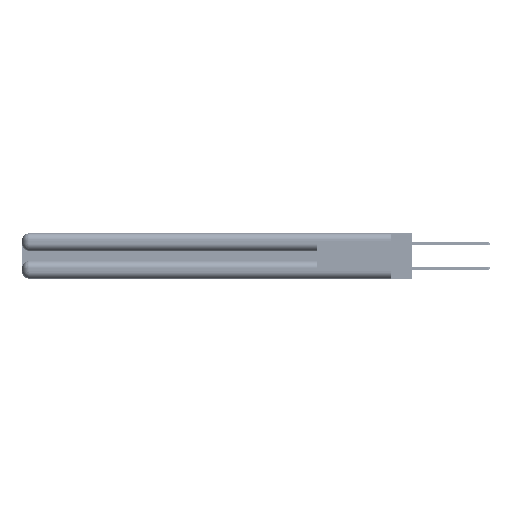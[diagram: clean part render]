
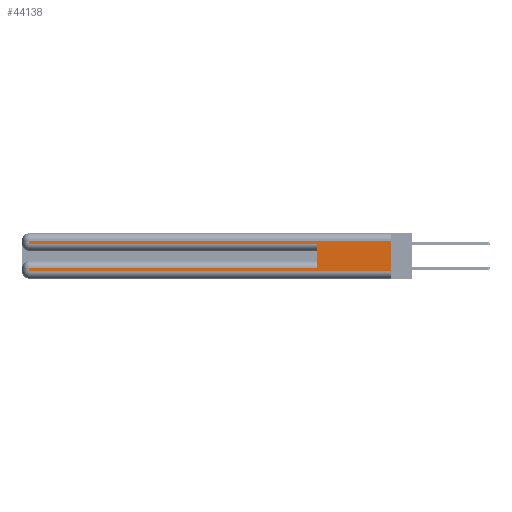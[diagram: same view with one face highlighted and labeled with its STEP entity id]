
A CAD part, left-side view. The second image highlights one B-rep face of the part: STEP entity #44138.
In plain terms, the highlighted planar face has unit normal (-1, 0, 0).
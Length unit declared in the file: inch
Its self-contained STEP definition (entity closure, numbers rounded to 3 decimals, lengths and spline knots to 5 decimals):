
#1636 = CARTESIAN_POINT ( 'NONE',  ( 0., 0., 0.37 ) ) ;
#1816 = CARTESIAN_POINT ( 'NONE',  ( 0., 0., 0.37 ) ) ;
#1879 = VERTEX_POINT ( 'NONE', #38098 ) ;
#2134 = DIRECTION ( 'NONE',  ( 0., 0., -1. ) ) ;
#2666 = ORIENTED_EDGE ( 'NONE', *, *, #47249, .T. ) ;
#5046 = LINE ( 'NONE', #14562, #25604 ) ;
#6629 = DIRECTION ( 'NONE',  ( 0., -1., 0. ) ) ;
#7760 = EDGE_CURVE ( 'NONE', #37095, #1879, #13730, .T. ) ;
#7888 = CARTESIAN_POINT ( 'NONE',  ( 0., 0., 0.06 ) ) ;
#8126 = DIRECTION ( 'NONE',  ( 0., 0., 1. ) ) ;
#9948 = CARTESIAN_POINT ( 'NONE',  ( 0., 2.94, 0.37 ) ) ;
#10549 = CARTESIAN_POINT ( 'NONE',  ( 0., 2.94, 0.31 ) ) ;
#12136 = VECTOR ( 'NONE', #12455, 39.37008 ) ;
#12435 = ORIENTED_EDGE ( 'NONE', *, *, #36582, .T. ) ;
#12455 = DIRECTION ( 'NONE',  ( 0., 1., 0. ) ) ;
#12641 = CARTESIAN_POINT ( 'NONE',  ( 0., 0.6, 0.145 ) ) ;
#13730 = LINE ( 'NONE', #9948, #21388 ) ;
#14257 = DIRECTION ( 'NONE',  ( 0., 0., -1. ) ) ;
#14562 = CARTESIAN_POINT ( 'NONE',  ( 0., 0., 0.06 ) ) ;
#18042 = DIRECTION ( 'NONE',  ( 0., -1., 0. ) ) ;
#18179 = DIRECTION ( 'NONE',  ( 0., 0., -1. ) ) ;
#18964 = CARTESIAN_POINT ( 'NONE',  ( 0., 2.94, 0.285 ) ) ;
#19004 = FACE_OUTER_BOUND ( 'NONE', #50883, .T. ) ;
#21388 = VECTOR ( 'NONE', #18179, 39.37008 ) ;
#21871 = EDGE_CURVE ( 'NONE', #32762, #28467, #35847, .T. ) ;
#23206 = LINE ( 'NONE', #50889, #35406 ) ;
#24456 = VECTOR ( 'NONE', #8126, 39.37008 ) ;
#24737 = VERTEX_POINT ( 'NONE', #26861 ) ;
#25323 = EDGE_CURVE ( 'NONE', #25423, #47871, #34207, .T. ) ;
#25423 = VERTEX_POINT ( 'NONE', #47797 ) ;
#25604 = VECTOR ( 'NONE', #6629, 39.37008 ) ;
#26383 = ORIENTED_EDGE ( 'NONE', *, *, #41433, .F. ) ;
#26861 = CARTESIAN_POINT ( 'NONE',  ( 0., 0.6, 0.085 ) ) ;
#28196 = CARTESIAN_POINT ( 'NONE',  ( 0., 0., 0.31 ) ) ;
#28467 = VERTEX_POINT ( 'NONE', #18964 ) ;
#30364 = DIRECTION ( 'NONE',  ( 0., 0., -1. ) ) ;
#32016 = ORIENTED_EDGE ( 'NONE', *, *, #40939, .T. ) ;
#32537 = DIRECTION ( 'NONE',  ( 0., 1., 0. ) ) ;
#32762 = VERTEX_POINT ( 'NONE', #10549 ) ;
#33810 = ORIENTED_EDGE ( 'NONE', *, *, #25323, .F. ) ;
#34207 = LINE ( 'NONE', #1636, #38074 ) ;
#34550 = VECTOR ( 'NONE', #2134, 39.37008 ) ;
#35192 = ORIENTED_EDGE ( 'NONE', *, *, #21871, .T. ) ;
#35406 = VECTOR ( 'NONE', #18042, 39.37008 ) ;
#35847 = LINE ( 'NONE', #38945, #34550 ) ;
#36582 = EDGE_CURVE ( 'NONE', #24737, #37095, #48229, .T. ) ;
#37095 = VERTEX_POINT ( 'NONE', #47975 ) ;
#38074 = VECTOR ( 'NONE', #30364, 39.37008 ) ;
#38098 = CARTESIAN_POINT ( 'NONE',  ( 0., 2.94, 0.06 ) ) ;
#38945 = CARTESIAN_POINT ( 'NONE',  ( 0., 2.94, 0.37 ) ) ;
#40939 = EDGE_CURVE ( 'NONE', #28467, #43204, #23206, .T. ) ;
#41433 = EDGE_CURVE ( 'NONE', #24737, #43204, #47607, .T. ) ;
#42919 = EDGE_CURVE ( 'NONE', #1879, #47871, #5046, .T. ) ;
#43124 = PLANE ( 'NONE',  #45474 ) ;
#43204 = VERTEX_POINT ( 'NONE', #44861 ) ;
#44138 = ADVANCED_FACE ( 'NONE', ( #19004 ), #43124, .F. ) ;
#44861 = CARTESIAN_POINT ( 'NONE',  ( 0., 0.6, 0.285 ) ) ;
#45337 = CARTESIAN_POINT ( 'NONE',  ( 0., 0., 0.085 ) ) ;
#45474 = AXIS2_PLACEMENT_3D ( 'NONE', #1816, #50675, #14257 ) ;
#47249 = EDGE_CURVE ( 'NONE', #25423, #32762, #52545, .T. ) ;
#47585 = VECTOR ( 'NONE', #32537, 39.37008 ) ;
#47607 = LINE ( 'NONE', #12641, #24456 ) ;
#47797 = CARTESIAN_POINT ( 'NONE',  ( 0., 0., 0.31 ) ) ;
#47871 = VERTEX_POINT ( 'NONE', #7888 ) ;
#47975 = CARTESIAN_POINT ( 'NONE',  ( 0., 2.94, 0.085 ) ) ;
#48229 = LINE ( 'NONE', #45337, #47585 ) ;
#48563 = ORIENTED_EDGE ( 'NONE', *, *, #7760, .T. ) ;
#50675 = DIRECTION ( 'NONE',  ( 1., 0., 0. ) ) ;
#50883 = EDGE_LOOP ( 'NONE', ( #33810, #2666, #35192, #32016, #26383, #12435, #48563, #51506 ) ) ;
#50889 = CARTESIAN_POINT ( 'NONE',  ( 0., 0., 0.285 ) ) ;
#51506 = ORIENTED_EDGE ( 'NONE', *, *, #42919, .T. ) ;
#52545 = LINE ( 'NONE', #28196, #12136 ) ;
